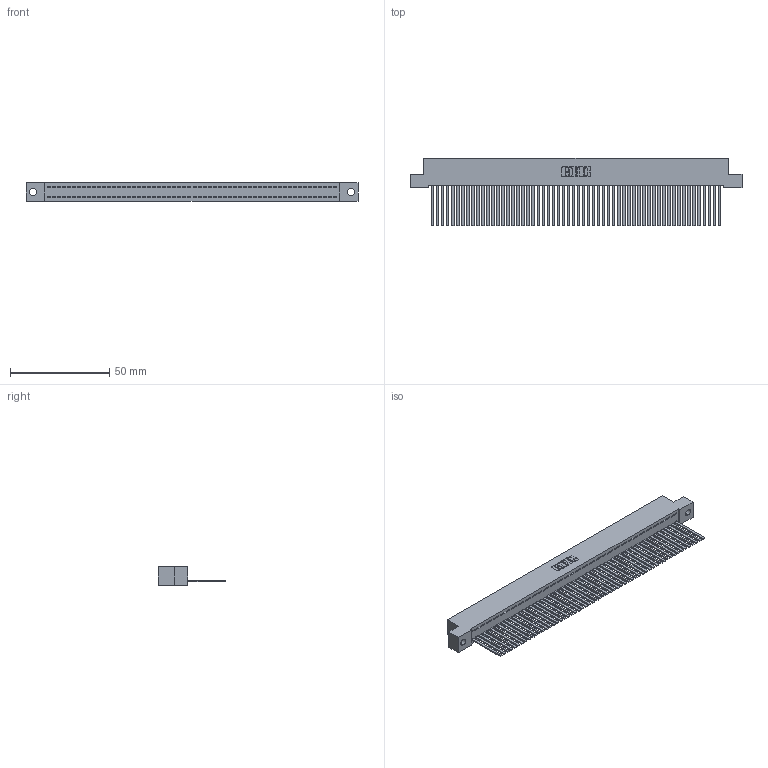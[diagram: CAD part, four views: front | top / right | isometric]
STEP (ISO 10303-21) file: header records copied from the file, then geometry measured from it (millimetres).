
FILE_DESCRIPTION (( 'STEP AP203' ), '1' );
FILE_NAME ('342-058-544-102.STEP', '2018-08-13T05:29:55', ( '' ), ( '' ), 'SwSTEP 2.0', 'SolidWorks 2016', '' );
FILE_SCHEMA (( 'CONFIG_CONTROL_DESIGN' ));
Length unit declared in the file: inch
Products named in the file (3): 342 Part_.128 Slot; 345-292-001_345-293-144; 342-058-544-102
Assembly tree (59 placements, depth 2):
  342-058-544-102
    342 Part_.128 Slot
    345-292-001_345-293-144  x58
Bounding box: 167.64 x 34.3 x 9.4 mm (x, y, z)
Volume: 15377.2 mm3; surface area: 24550.8 mm2
Topology: 59 solids, 59 shells, 3130 faces, 9475 edges, 6238 vertices
Faces by surface type: plane 2274, cylinder 856
Entity records: 33207 total; most frequent: CARTESIAN_POINT 5732, ORIENTED_EDGE 5726, DIRECTION 4799, EDGE_CURVE 2863, LINE 2739, VECTOR 2739, VERTEX_POINT 1906, AXIS2_PLACEMENT_3D 1030
